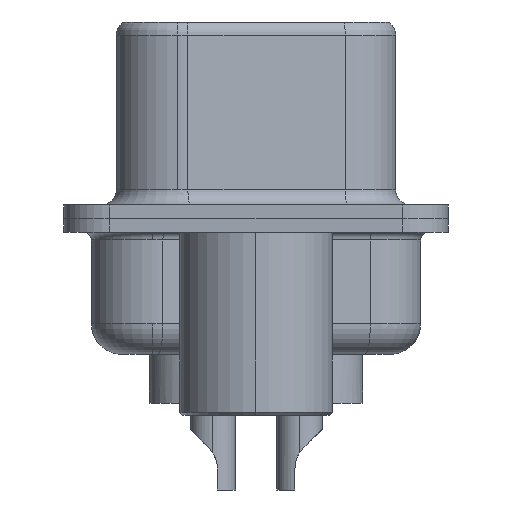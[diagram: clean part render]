
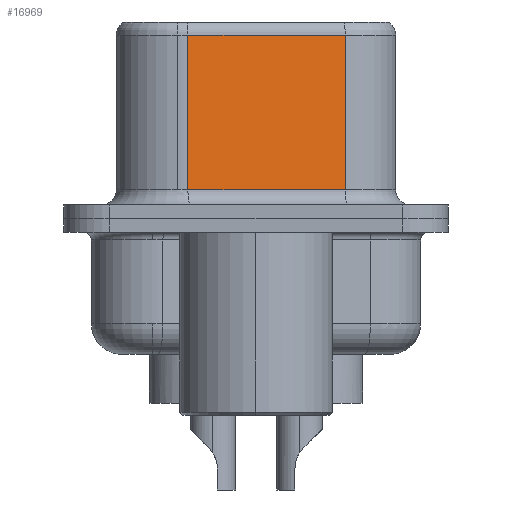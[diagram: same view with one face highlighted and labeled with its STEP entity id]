
A CAD part, left-side view. The second image highlights one B-rep face of the part: STEP entity #16969.
In plain terms, the highlighted planar face has unit normal (-0.985, -0.174, 0).
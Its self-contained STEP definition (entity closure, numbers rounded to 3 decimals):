
#1027 = VERTEX_POINT ( 'NONE', #4884 ) ;
#1368 = VECTOR ( 'NONE', #10661, 1000. ) ;
#1658 = VECTOR ( 'NONE', #4696, 1000. ) ;
#1829 = ORIENTED_EDGE ( 'NONE', *, *, #14664, .T. ) ;
#2714 = AXIS2_PLACEMENT_3D ( 'NONE', #5255, #9997, #14220 ) ;
#3236 = FACE_OUTER_BOUND ( 'NONE', #9713, .T. ) ;
#3264 = EDGE_CURVE ( 'NONE', #9666, #4364, #8432, .T. ) ;
#4364 = VERTEX_POINT ( 'NONE', #12926 ) ;
#4563 = CARTESIAN_POINT ( 'NONE',  ( 4.575, -2.927, 0.95 ) ) ;
#4696 = DIRECTION ( 'NONE',  ( 0., 0., -1. ) ) ;
#4884 = CARTESIAN_POINT ( 'NONE',  ( 3.665, 2.233, 6.02 ) ) ;
#5016 = ORIENTED_EDGE ( 'NONE', *, *, #5934, .T. ) ;
#5076 = ORIENTED_EDGE ( 'NONE', *, *, #9790, .T. ) ;
#5156 = CARTESIAN_POINT ( 'NONE',  ( 3.665, 2.233, 0.95 ) ) ;
#5255 = CARTESIAN_POINT ( 'NONE',  ( 4.575, -2.927, 6.52 ) ) ;
#5927 = LINE ( 'NONE', #4563, #1368 ) ;
#5934 = EDGE_CURVE ( 'NONE', #14924, #4364, #5927, .T. ) ;
#7644 = CARTESIAN_POINT ( 'NONE',  ( 4.575, -2.927, 6.02 ) ) ;
#8432 = LINE ( 'NONE', #19104, #18902 ) ;
#8593 = VECTOR ( 'NONE', #17255, 1000. ) ;
#9218 = PLANE ( 'NONE',  #2714 ) ;
#9666 = VERTEX_POINT ( 'NONE', #7644 ) ;
#9713 = EDGE_LOOP ( 'NONE', ( #14870, #1829, #5076, #5016 ) ) ;
#9790 = EDGE_CURVE ( 'NONE', #1027, #14924, #13353, .T. ) ;
#9997 = DIRECTION ( 'NONE',  ( 0.985, 0.174, 0. ) ) ;
#10661 = DIRECTION ( 'NONE',  ( 0.174, -0.985, 0. ) ) ;
#12926 = CARTESIAN_POINT ( 'NONE',  ( 4.575, -2.927, 0.95 ) ) ;
#13353 = LINE ( 'NONE', #13649, #1658 ) ;
#13649 = CARTESIAN_POINT ( 'NONE',  ( 3.665, 2.233, 6.52 ) ) ;
#14220 = DIRECTION ( 'NONE',  ( -0.174, 0.985, 0. ) ) ;
#14631 = CARTESIAN_POINT ( 'NONE',  ( 4.575, -2.927, 6.02 ) ) ;
#14664 = EDGE_CURVE ( 'NONE', #9666, #1027, #17351, .T. ) ;
#14870 = ORIENTED_EDGE ( 'NONE', *, *, #3264, .F. ) ;
#14924 = VERTEX_POINT ( 'NONE', #5156 ) ;
#16969 = ADVANCED_FACE ( 'NONE', ( #3236 ), #9218, .F. ) ;
#17255 = DIRECTION ( 'NONE',  ( -0.174, 0.985, 0. ) ) ;
#17351 = LINE ( 'NONE', #14631, #8593 ) ;
#18902 = VECTOR ( 'NONE', #19200, 1000. ) ;
#19104 = CARTESIAN_POINT ( 'NONE',  ( 4.575, -2.927, 6.52 ) ) ;
#19200 = DIRECTION ( 'NONE',  ( 0., 0., -1. ) ) ;
